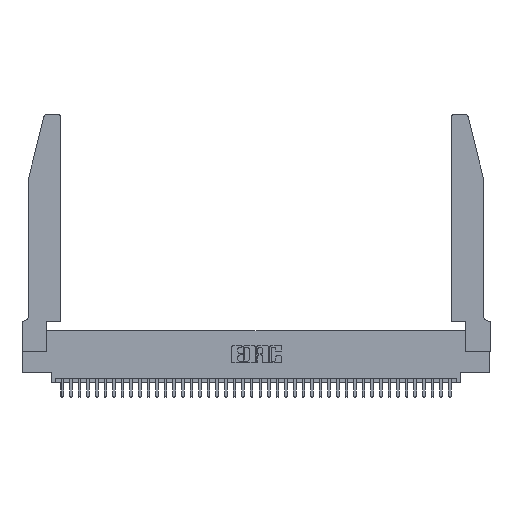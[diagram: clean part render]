
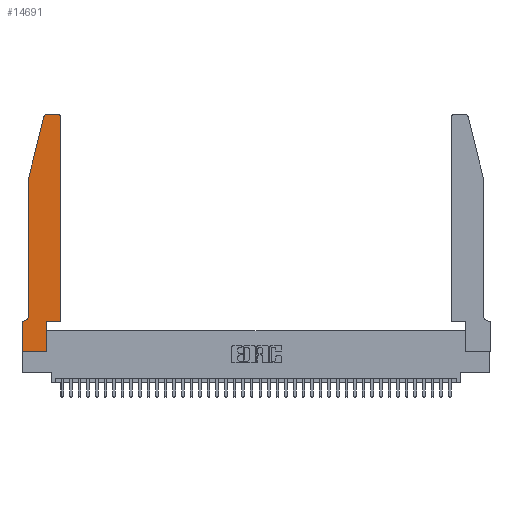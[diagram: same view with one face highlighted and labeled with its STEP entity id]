
A CAD part, top view. The second image highlights one B-rep face of the part: STEP entity #14691.
In plain terms, the highlighted planar face has unit normal (0, 0, 1).
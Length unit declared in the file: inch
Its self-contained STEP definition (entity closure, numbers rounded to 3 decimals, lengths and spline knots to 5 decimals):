
#414 = LINE ( 'NONE', #1845, #1403 ) ;
#1010 = VECTOR ( 'NONE', #32541, 39.37008 ) ;
#1176 = CARTESIAN_POINT ( 'NONE',  ( 0.4505, 0.35, 0.37 ) ) ;
#1216 = ORIENTED_EDGE ( 'NONE', *, *, #35927, .T. ) ;
#1403 = VECTOR ( 'NONE', #20776, 39.37008 ) ;
#1700 = VECTOR ( 'NONE', #27472, 39.37008 ) ;
#1784 = CARTESIAN_POINT ( 'NONE',  ( 0.4505, 2.72, 0.37 ) ) ;
#1845 = CARTESIAN_POINT ( 'NONE',  ( 0., 0., 0.37 ) ) ;
#2042 = LINE ( 'NONE', #7228, #25257 ) ;
#2097 = VERTEX_POINT ( 'NONE', #20916 ) ;
#2509 = LINE ( 'NONE', #25899, #26707 ) ;
#2750 = ORIENTED_EDGE ( 'NONE', *, *, #9028, .T. ) ;
#2829 = EDGE_CURVE ( 'NONE', #33514, #39588, #9391, .T. ) ;
#3399 = EDGE_CURVE ( 'NONE', #38726, #13721, #3499, .T. ) ;
#3430 = EDGE_CURVE ( 'NONE', #35649, #12701, #2509, .T. ) ;
#3499 = LINE ( 'NONE', #3798, #11939 ) ;
#3798 = CARTESIAN_POINT ( 'NONE',  ( 0.2865, 0.35, 0.37 ) ) ;
#4063 = DIRECTION ( 'NONE',  ( 0., 0., 1. ) ) ;
#4381 = DIRECTION ( 'NONE',  ( 0., 0., 1. ) ) ;
#4473 = DIRECTION ( 'NONE',  ( 0., -1., 0. ) ) ;
#5404 = CARTESIAN_POINT ( 'NONE',  ( 0., 0., 0.37 ) ) ;
#5599 = CARTESIAN_POINT ( 'NONE',  ( 0.4505, 0.35, 0.37 ) ) ;
#7070 = EDGE_CURVE ( 'NONE', #39588, #35869, #36983, .T. ) ;
#7228 = CARTESIAN_POINT ( 'NONE',  ( 0.4505, 0.35, 0.37 ) ) ;
#7323 = CARTESIAN_POINT ( 'NONE',  ( 0.284, 2.72, 0.37 ) ) ;
#8338 = EDGE_CURVE ( 'NONE', #18876, #22587, #13055, .T. ) ;
#8782 = DIRECTION ( 'NONE',  ( 0., 1., 0. ) ) ;
#8912 = CARTESIAN_POINT ( 'NONE',  ( 0.0055, 0.42, 0.37 ) ) ;
#9028 = EDGE_CURVE ( 'NONE', #31092, #35649, #28240, .T. ) ;
#9391 = LINE ( 'NONE', #29462, #1010 ) ;
#10385 = CARTESIAN_POINT ( 'NONE',  ( 0.25487, 2.72718, 0.37 ) ) ;
#10528 = DIRECTION ( 'NONE',  ( 1., 0., 0. ) ) ;
#11017 = VERTEX_POINT ( 'NONE', #1176 ) ;
#11939 = VECTOR ( 'NONE', #22736, 39.37008 ) ;
#11995 = ORIENTED_EDGE ( 'NONE', *, *, #3399, .T. ) ;
#12117 = DIRECTION ( 'NONE',  ( -1., 0., 0. ) ) ;
#12683 = CARTESIAN_POINT ( 'NONE',  ( 0.284, 2.75, 0.37 ) ) ;
#12701 = VERTEX_POINT ( 'NONE', #12683 ) ;
#13055 = LINE ( 'NONE', #38748, #28785 ) ;
#13350 = DIRECTION ( 'NONE',  ( -1., 0., 0. ) ) ;
#13699 = AXIS2_PLACEMENT_3D ( 'NONE', #8912, #30863, #12117 ) ;
#13721 = VERTEX_POINT ( 'NONE', #14389 ) ;
#14389 = CARTESIAN_POINT ( 'NONE',  ( 0.2865, 0.35, 0.37 ) ) ;
#14392 = ORIENTED_EDGE ( 'NONE', *, *, #2829, .T. ) ;
#14691 = ADVANCED_FACE ( 'NONE', ( #35210 ), #35606, .T. ) ;
#15090 = ORIENTED_EDGE ( 'NONE', *, *, #17454, .T. ) ;
#15474 = CARTESIAN_POINT ( 'NONE',  ( 0.2865, 0., 0.37 ) ) ;
#15567 = VECTOR ( 'NONE', #8782, 39.37008 ) ;
#17110 = ORIENTED_EDGE ( 'NONE', *, *, #20709, .T. ) ;
#17454 = EDGE_CURVE ( 'NONE', #2097, #38726, #414, .T. ) ;
#18876 = VERTEX_POINT ( 'NONE', #23248 ) ;
#19316 = ORIENTED_EDGE ( 'NONE', *, *, #20350, .T. ) ;
#19662 = CARTESIAN_POINT ( 'NONE',  ( 0.0755, 0.42, 0.37 ) ) ;
#19939 = AXIS2_PLACEMENT_3D ( 'NONE', #32521, #4381, #26463 ) ;
#19958 = DIRECTION ( 'NONE',  ( 1., 0., 0. ) ) ;
#20342 = EDGE_CURVE ( 'NONE', #11017, #31092, #32194, .T. ) ;
#20350 = EDGE_CURVE ( 'NONE', #35869, #18876, #22968, .T. ) ;
#20709 = EDGE_CURVE ( 'NONE', #22587, #2097, #25888, .T. ) ;
#20776 = DIRECTION ( 'NONE',  ( 1., 0., 0. ) ) ;
#20916 = CARTESIAN_POINT ( 'NONE',  ( 0., 0., 0.37 ) ) ;
#22341 = EDGE_CURVE ( 'NONE', #13721, #11017, #2042, .T. ) ;
#22370 = ORIENTED_EDGE ( 'NONE', *, *, #20342, .T. ) ;
#22587 = VERTEX_POINT ( 'NONE', #33644 ) ;
#22736 = DIRECTION ( 'NONE',  ( 0., 1., 0. ) ) ;
#22968 = CIRCLE ( 'NONE', #13699, 0.07 ) ;
#23004 = CARTESIAN_POINT ( 'NONE',  ( 0.4205, 2.72, 0.37 ) ) ;
#23248 = CARTESIAN_POINT ( 'NONE',  ( 0.0055, 0.35, 0.37 ) ) ;
#23312 = DIRECTION ( 'NONE',  ( -1., 0., 0. ) ) ;
#24644 = ORIENTED_EDGE ( 'NONE', *, *, #3430, .T. ) ;
#24901 = CARTESIAN_POINT ( 'NONE',  ( 0.4205, 2.75, 0.37 ) ) ;
#25257 = VECTOR ( 'NONE', #19958, 39.37008 ) ;
#25888 = LINE ( 'NONE', #5404, #1700 ) ;
#25899 = CARTESIAN_POINT ( 'NONE',  ( 0.2605, 2.75, 0.37 ) ) ;
#26092 = ORIENTED_EDGE ( 'NONE', *, *, #8338, .T. ) ;
#26144 = DIRECTION ( 'NONE',  ( 1., 0., 0. ) ) ;
#26463 = DIRECTION ( 'NONE',  ( 1., 0., 0. ) ) ;
#26707 = VECTOR ( 'NONE', #13350, 39.37008 ) ;
#26916 = AXIS2_PLACEMENT_3D ( 'NONE', #23004, #4063, #26144 ) ;
#27472 = DIRECTION ( 'NONE',  ( 0., -1., 0. ) ) ;
#28240 = CIRCLE ( 'NONE', #26916, 0.03 ) ;
#28731 = CARTESIAN_POINT ( 'NONE',  ( 0.0755, 2., 0.37 ) ) ;
#28785 = VECTOR ( 'NONE', #23312, 39.37008 ) ;
#28817 = VECTOR ( 'NONE', #4473, 39.37008 ) ;
#29364 = DIRECTION ( 'NONE',  ( 0., 0., 1. ) ) ;
#29462 = CARTESIAN_POINT ( 'NONE',  ( 0.0755, 2., 0.37 ) ) ;
#30863 = DIRECTION ( 'NONE',  ( 0., 0., -1. ) ) ;
#31092 = VERTEX_POINT ( 'NONE', #1784 ) ;
#32194 = LINE ( 'NONE', #5599, #15567 ) ;
#32360 = EDGE_LOOP ( 'NONE', ( #24644, #1216, #14392, #37404, #19316, #26092, #17110, #15090, #11995, #40246, #22370, #2750 ) ) ;
#32521 = CARTESIAN_POINT ( 'NONE',  ( 0., 0.35, 0.37 ) ) ;
#32541 = DIRECTION ( 'NONE',  ( -0.239, -0.971, 0. ) ) ;
#33514 = VERTEX_POINT ( 'NONE', #10385 ) ;
#33644 = CARTESIAN_POINT ( 'NONE',  ( 0., 0.35, 0.37 ) ) ;
#35210 = FACE_OUTER_BOUND ( 'NONE', #32360, .T. ) ;
#35606 = PLANE ( 'NONE',  #19939 ) ;
#35649 = VERTEX_POINT ( 'NONE', #24901 ) ;
#35683 = CARTESIAN_POINT ( 'NONE',  ( 0.0755, 2., 0.37 ) ) ;
#35869 = VERTEX_POINT ( 'NONE', #19662 ) ;
#35927 = EDGE_CURVE ( 'NONE', #12701, #33514, #37251, .T. ) ;
#36983 = LINE ( 'NONE', #35683, #28817 ) ;
#37251 = CIRCLE ( 'NONE', #39571, 0.03 ) ;
#37404 = ORIENTED_EDGE ( 'NONE', *, *, #7070, .T. ) ;
#38726 = VERTEX_POINT ( 'NONE', #15474 ) ;
#38748 = CARTESIAN_POINT ( 'NONE',  ( 0.0755, 0.35, 0.37 ) ) ;
#39571 = AXIS2_PLACEMENT_3D ( 'NONE', #7323, #29364, #10528 ) ;
#39588 = VERTEX_POINT ( 'NONE', #28731 ) ;
#40246 = ORIENTED_EDGE ( 'NONE', *, *, #22341, .T. ) ;
